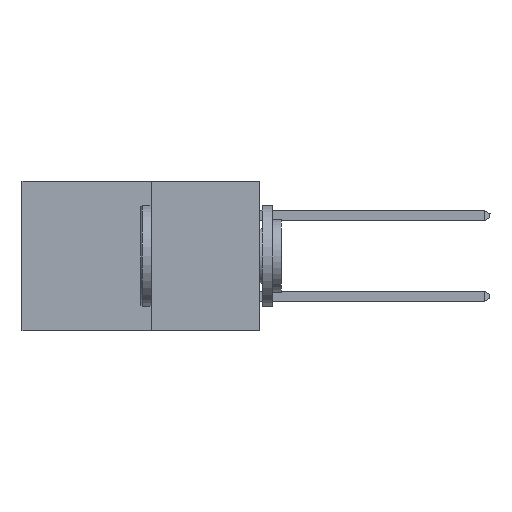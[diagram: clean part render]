
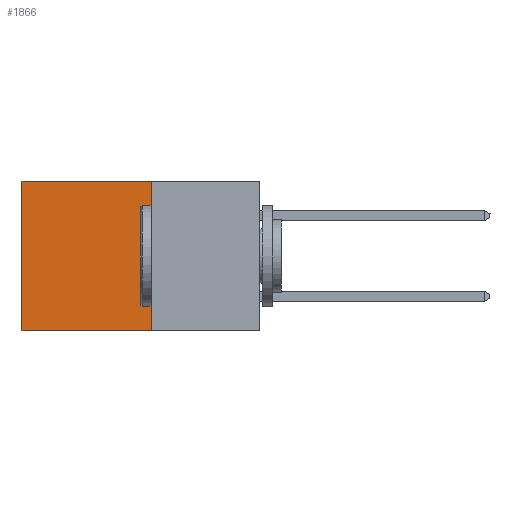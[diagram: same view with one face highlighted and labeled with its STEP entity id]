
A CAD part, left-side view. The second image highlights one B-rep face of the part: STEP entity #1866.
In plain terms, the highlighted planar face has unit normal (-1, 0, 0).
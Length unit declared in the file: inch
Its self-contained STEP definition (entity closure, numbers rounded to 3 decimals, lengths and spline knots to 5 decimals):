
#212 = VECTOR ( 'NONE', #1678, 39.37008 ) ;
#537 = VERTEX_POINT ( 'NONE', #12460 ) ;
#1111 = EDGE_CURVE ( 'NONE', #15421, #11603, #4019, .T. ) ;
#1165 = EDGE_CURVE ( 'NONE', #15421, #537, #9561, .T. ) ;
#1577 = CARTESIAN_POINT ( 'NONE',  ( 0.277, 0.59, -0.37 ) ) ;
#1678 = DIRECTION ( 'NONE',  ( 0., 1., 0. ) ) ;
#1866 = ADVANCED_FACE ( 'NONE', ( #15407 ), #8797, .F. ) ;
#3005 = EDGE_CURVE ( 'NONE', #537, #12782, #9338, .T. ) ;
#3998 = CARTESIAN_POINT ( 'NONE',  ( 0.277, 0.59, 0. ) ) ;
#4019 = LINE ( 'NONE', #12005, #212 ) ;
#5375 = ORIENTED_EDGE ( 'NONE', *, *, #1165, .F. ) ;
#5964 = AXIS2_PLACEMENT_3D ( 'NONE', #13616, #13531, #9050 ) ;
#6823 = ORIENTED_EDGE ( 'NONE', *, *, #3005, .F. ) ;
#6949 = VECTOR ( 'NONE', #14192, 39.37008 ) ;
#7641 = DIRECTION ( 'NONE',  ( 0., 0., -1. ) ) ;
#8753 = EDGE_LOOP ( 'NONE', ( #14829, #6823, #5375, #14948 ) ) ;
#8797 = PLANE ( 'NONE',  #5964 ) ;
#9050 = DIRECTION ( 'NONE',  ( 0., 0., -1. ) ) ;
#9228 = CARTESIAN_POINT ( 'NONE',  ( 0.277, 0.59, -0.37 ) ) ;
#9338 = LINE ( 'NONE', #15449, #13062 ) ;
#9561 = LINE ( 'NONE', #13132, #15771 ) ;
#10285 = LINE ( 'NONE', #1577, #6949 ) ;
#11603 = VERTEX_POINT ( 'NONE', #3998 ) ;
#12005 = CARTESIAN_POINT ( 'NONE',  ( 0.277, 0.27, 0. ) ) ;
#12460 = CARTESIAN_POINT ( 'NONE',  ( 0.277, 0.27, -0.37 ) ) ;
#12782 = VERTEX_POINT ( 'NONE', #9228 ) ;
#12948 = CARTESIAN_POINT ( 'NONE',  ( 0.277, 0.27, 0. ) ) ;
#13062 = VECTOR ( 'NONE', #15984, 39.37008 ) ;
#13132 = CARTESIAN_POINT ( 'NONE',  ( 0.277, 0.27, -0.37 ) ) ;
#13531 = DIRECTION ( 'NONE',  ( 1., 0., 0. ) ) ;
#13616 = CARTESIAN_POINT ( 'NONE',  ( 0.277, 0.27, -0.37 ) ) ;
#14192 = DIRECTION ( 'NONE',  ( 0., 0., -1. ) ) ;
#14829 = ORIENTED_EDGE ( 'NONE', *, *, #15419, .T. ) ;
#14948 = ORIENTED_EDGE ( 'NONE', *, *, #1111, .T. ) ;
#15407 = FACE_OUTER_BOUND ( 'NONE', #8753, .T. ) ;
#15419 = EDGE_CURVE ( 'NONE', #11603, #12782, #10285, .T. ) ;
#15421 = VERTEX_POINT ( 'NONE', #12948 ) ;
#15449 = CARTESIAN_POINT ( 'NONE',  ( 0.277, 0.27, -0.37 ) ) ;
#15771 = VECTOR ( 'NONE', #7641, 39.37008 ) ;
#15984 = DIRECTION ( 'NONE',  ( 0., 1., 0. ) ) ;
